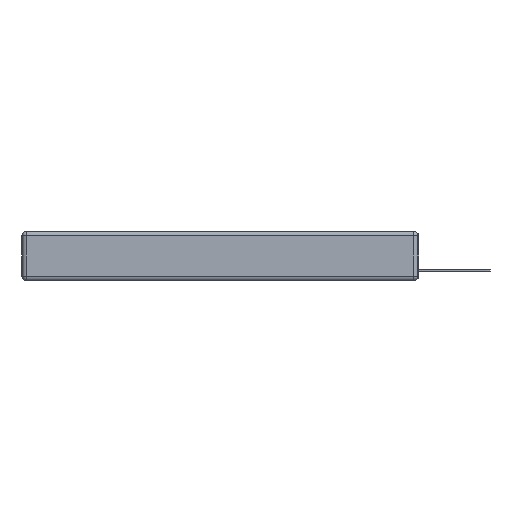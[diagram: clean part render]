
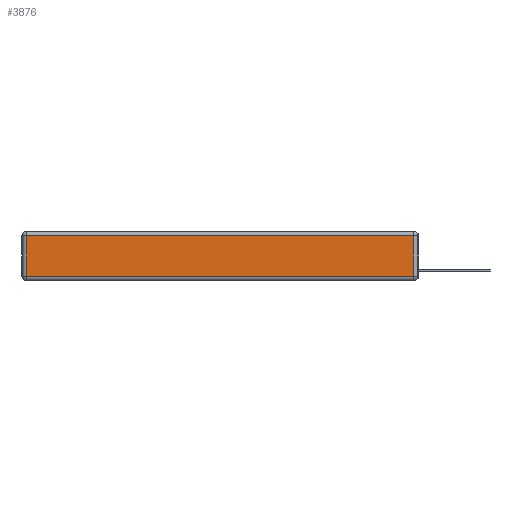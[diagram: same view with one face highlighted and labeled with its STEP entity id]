
A CAD part, left-side view. The second image highlights one B-rep face of the part: STEP entity #3876.
In plain terms, the highlighted planar face has unit normal (-1, 0, 0).
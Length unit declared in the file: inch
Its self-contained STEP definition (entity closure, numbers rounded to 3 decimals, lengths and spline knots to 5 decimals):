
#1442 = ORIENTED_EDGE ( 'NONE', *, *, #21552, .T. ) ;
#3115 = VECTOR ( 'NONE', #9001, 39.37008 ) ;
#3150 = CARTESIAN_POINT ( 'NONE',  ( 0., 0., -0.343 ) ) ;
#3876 = ADVANCED_FACE ( 'NONE', ( #5884 ), #5377, .T. ) ;
#3994 = EDGE_CURVE ( 'NONE', #8763, #8343, #9489, .T. ) ;
#5377 = PLANE ( 'NONE',  #6548 ) ;
#5617 = CARTESIAN_POINT ( 'NONE',  ( 0., 0.03, -0.03 ) ) ;
#5884 = FACE_OUTER_BOUND ( 'NONE', #11015, .T. ) ;
#6548 = AXIS2_PLACEMENT_3D ( 'NONE', #3150, #8723, #12605 ) ;
#6766 = CARTESIAN_POINT ( 'NONE',  ( 0., 0., -0.313 ) ) ;
#8343 = VERTEX_POINT ( 'NONE', #5617 ) ;
#8723 = DIRECTION ( 'NONE',  ( -1., 0., 0. ) ) ;
#8763 = VERTEX_POINT ( 'NONE', #20171 ) ;
#9001 = DIRECTION ( 'NONE',  ( 0., 0., -1. ) ) ;
#9489 = LINE ( 'NONE', #14680, #24219 ) ;
#9964 = VECTOR ( 'NONE', #12830, 39.37008 ) ;
#10597 = LINE ( 'NONE', #12976, #3115 ) ;
#10803 = DIRECTION ( 'NONE',  ( 0., 0., 1. ) ) ;
#11015 = EDGE_LOOP ( 'NONE', ( #15415, #19837, #17413, #1442 ) ) ;
#11155 = CARTESIAN_POINT ( 'NONE',  ( 0., 2.75, -0.03 ) ) ;
#12605 = DIRECTION ( 'NONE',  ( 0., 0., 1. ) ) ;
#12830 = DIRECTION ( 'NONE',  ( 0., 1., 0. ) ) ;
#12976 = CARTESIAN_POINT ( 'NONE',  ( 0., 2.72, -0.343 ) ) ;
#13265 = VERTEX_POINT ( 'NONE', #22820 ) ;
#13976 = CARTESIAN_POINT ( 'NONE',  ( 0., 2.72, -0.03 ) ) ;
#14126 = VERTEX_POINT ( 'NONE', #13976 ) ;
#14680 = CARTESIAN_POINT ( 'NONE',  ( 0., 0.03, -0.343 ) ) ;
#15415 = ORIENTED_EDGE ( 'NONE', *, *, #21964, .T. ) ;
#16555 = DIRECTION ( 'NONE',  ( 0., -1., 0. ) ) ;
#17413 = ORIENTED_EDGE ( 'NONE', *, *, #22009, .T. ) ;
#19038 = VECTOR ( 'NONE', #16555, 39.37008 ) ;
#19837 = ORIENTED_EDGE ( 'NONE', *, *, #3994, .T. ) ;
#20171 = CARTESIAN_POINT ( 'NONE',  ( 0., 0.03, -0.313 ) ) ;
#21404 = LINE ( 'NONE', #6766, #19038 ) ;
#21552 = EDGE_CURVE ( 'NONE', #14126, #13265, #10597, .T. ) ;
#21690 = LINE ( 'NONE', #11155, #9964 ) ;
#21964 = EDGE_CURVE ( 'NONE', #13265, #8763, #21404, .T. ) ;
#22009 = EDGE_CURVE ( 'NONE', #8343, #14126, #21690, .T. ) ;
#22820 = CARTESIAN_POINT ( 'NONE',  ( 0., 2.72, -0.313 ) ) ;
#24219 = VECTOR ( 'NONE', #10803, 39.37008 ) ;
